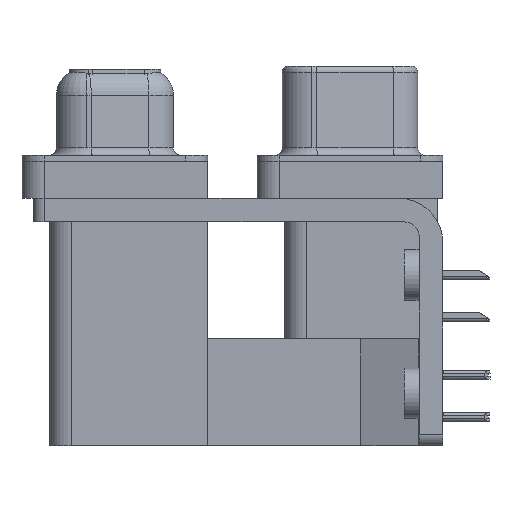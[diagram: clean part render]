
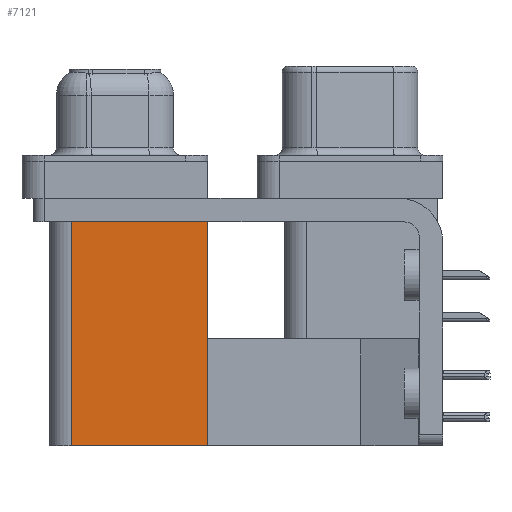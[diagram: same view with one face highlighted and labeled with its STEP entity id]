
A CAD part, left-side view. The second image highlights one B-rep face of the part: STEP entity #7121.
In plain terms, the highlighted planar face has unit normal (-1, 0, 0).
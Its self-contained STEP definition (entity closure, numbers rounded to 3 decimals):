
#9 = DIRECTION ( 'NONE',  ( 0., 1., 0. ) ) ;
#376 = CARTESIAN_POINT ( 'NONE',  ( 3.79, 9.6, -19.2 ) ) ;
#1913 = DIRECTION ( 'NONE',  ( 0., 0., 1. ) ) ;
#2137 = EDGE_CURVE ( 'NONE', #9776, #23284, #35572, .T. ) ;
#4661 = DIRECTION ( 'NONE',  ( 1., 0., 0. ) ) ;
#5410 = VECTOR ( 'NONE', #1913, 1000. ) ;
#6409 = VECTOR ( 'NONE', #9, 1000. ) ;
#6839 = EDGE_CURVE ( 'NONE', #23284, #26641, #33728, .T. ) ;
#7121 = ADVANCED_FACE ( 'NONE', ( #12788 ), #9567, .F. ) ;
#7362 = LINE ( 'NONE', #13041, #5410 ) ;
#9567 = PLANE ( 'NONE',  #13743 ) ;
#9776 = VERTEX_POINT ( 'NONE', #30247 ) ;
#10206 = CARTESIAN_POINT ( 'NONE',  ( 3.79, 9.6, -2.5 ) ) ;
#10513 = ORIENTED_EDGE ( 'NONE', *, *, #6839, .F. ) ;
#10575 = ORIENTED_EDGE ( 'NONE', *, *, #11053, .T. ) ;
#10929 = CARTESIAN_POINT ( 'NONE',  ( 3.79, 18.8, -19.2 ) ) ;
#11041 = EDGE_CURVE ( 'NONE', #9776, #22375, #7362, .T. ) ;
#11053 = EDGE_CURVE ( 'NONE', #22375, #26641, #16049, .T. ) ;
#12788 = FACE_OUTER_BOUND ( 'NONE', #20627, .T. ) ;
#13041 = CARTESIAN_POINT ( 'NONE',  ( 3.79, 9.6, -19.2 ) ) ;
#13743 = AXIS2_PLACEMENT_3D ( 'NONE', #27312, #4661, #26937 ) ;
#16049 = LINE ( 'NONE', #10206, #21660 ) ;
#17928 = VECTOR ( 'NONE', #19771, 1000. ) ;
#19331 = ORIENTED_EDGE ( 'NONE', *, *, #11041, .T. ) ;
#19771 = DIRECTION ( 'NONE',  ( 0., 0., 1. ) ) ;
#20420 = CARTESIAN_POINT ( 'NONE',  ( 3.79, 18.8, -2.5 ) ) ;
#20627 = EDGE_LOOP ( 'NONE', ( #10575, #10513, #31794, #19331 ) ) ;
#21660 = VECTOR ( 'NONE', #21710, 1000. ) ;
#21710 = DIRECTION ( 'NONE',  ( 0., 1., 0. ) ) ;
#22375 = VERTEX_POINT ( 'NONE', #28946 ) ;
#23284 = VERTEX_POINT ( 'NONE', #34696 ) ;
#26641 = VERTEX_POINT ( 'NONE', #20420 ) ;
#26937 = DIRECTION ( 'NONE',  ( 0., 1., 0. ) ) ;
#27312 = CARTESIAN_POINT ( 'NONE',  ( 3.79, 9.6, -19.2 ) ) ;
#28946 = CARTESIAN_POINT ( 'NONE',  ( 3.79, 9.6, -2.5 ) ) ;
#30247 = CARTESIAN_POINT ( 'NONE',  ( 3.79, 9.6, -19.2 ) ) ;
#31794 = ORIENTED_EDGE ( 'NONE', *, *, #2137, .F. ) ;
#33728 = LINE ( 'NONE', #10929, #17928 ) ;
#34696 = CARTESIAN_POINT ( 'NONE',  ( 3.79, 18.8, -19.2 ) ) ;
#35572 = LINE ( 'NONE', #376, #6409 ) ;
